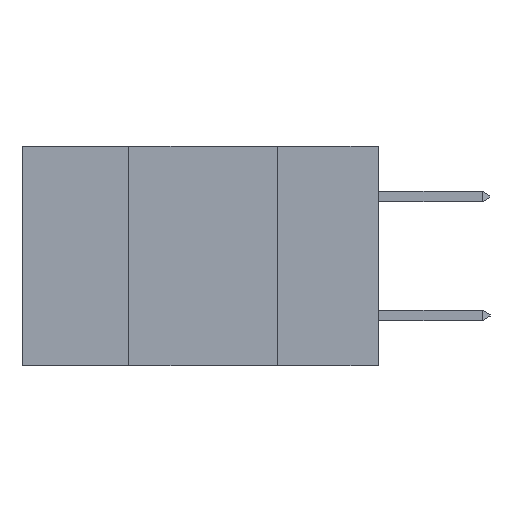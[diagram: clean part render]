
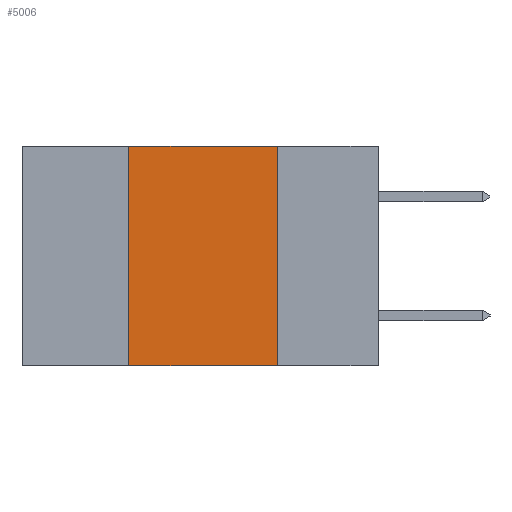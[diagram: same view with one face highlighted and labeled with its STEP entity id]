
A CAD part, left-side view. The second image highlights one B-rep face of the part: STEP entity #5006.
In plain terms, the highlighted planar face has unit normal (-1, 0, 0).
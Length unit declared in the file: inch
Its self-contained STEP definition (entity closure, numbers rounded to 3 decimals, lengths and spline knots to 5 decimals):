
#639 = CARTESIAN_POINT ( 'NONE',  ( 0., 0.17, 0. ) ) ;
#1431 = VECTOR ( 'NONE', #6552, 39.37008 ) ;
#1481 = DIRECTION ( 'NONE',  ( 0., -1., 0. ) ) ;
#1572 = CARTESIAN_POINT ( 'NONE',  ( 0., 0.42, -0.37 ) ) ;
#1961 = VERTEX_POINT ( 'NONE', #10551 ) ;
#2217 = ORIENTED_EDGE ( 'NONE', *, *, #4929, .T. ) ;
#2484 = CARTESIAN_POINT ( 'NONE',  ( 0., 0.17, -0.37 ) ) ;
#2720 = EDGE_CURVE ( 'NONE', #11193, #2944, #4649, .T. ) ;
#2770 = LINE ( 'NONE', #5174, #10688 ) ;
#2944 = VERTEX_POINT ( 'NONE', #2484 ) ;
#3335 = VERTEX_POINT ( 'NONE', #1572 ) ;
#3726 = CARTESIAN_POINT ( 'NONE',  ( 0., 0.42, -0.37 ) ) ;
#3785 = DIRECTION ( 'NONE',  ( 0., 0., -1. ) ) ;
#3831 = DIRECTION ( 'NONE',  ( 1., 0., 0. ) ) ;
#4030 = CARTESIAN_POINT ( 'NONE',  ( 0., 0.6, 0. ) ) ;
#4129 = PLANE ( 'NONE',  #8457 ) ;
#4649 = LINE ( 'NONE', #6662, #1431 ) ;
#4929 = EDGE_CURVE ( 'NONE', #3335, #2944, #2770, .T. ) ;
#4952 = DIRECTION ( 'NONE',  ( 0., -1., 0. ) ) ;
#5006 = ADVANCED_FACE ( 'NONE', ( #13049 ), #4129, .F. ) ;
#5174 = CARTESIAN_POINT ( 'NONE',  ( 0., 0.6, -0.37 ) ) ;
#6552 = DIRECTION ( 'NONE',  ( 0., 0., -1. ) ) ;
#6593 = VECTOR ( 'NONE', #11952, 39.37008 ) ;
#6662 = CARTESIAN_POINT ( 'NONE',  ( 0., 0.17, -0.37 ) ) ;
#7306 = VECTOR ( 'NONE', #1481, 39.37008 ) ;
#8457 = AXIS2_PLACEMENT_3D ( 'NONE', #4030, #3831, #3785 ) ;
#8822 = CARTESIAN_POINT ( 'NONE',  ( 0., 0.6, 0. ) ) ;
#9291 = LINE ( 'NONE', #3726, #6593 ) ;
#9820 = EDGE_CURVE ( 'NONE', #1961, #11193, #12464, .T. ) ;
#10148 = ORIENTED_EDGE ( 'NONE', *, *, #2720, .F. ) ;
#10278 = ORIENTED_EDGE ( 'NONE', *, *, #9820, .F. ) ;
#10551 = CARTESIAN_POINT ( 'NONE',  ( 0., 0.42, 0. ) ) ;
#10688 = VECTOR ( 'NONE', #4952, 39.37008 ) ;
#10907 = EDGE_LOOP ( 'NONE', ( #10148, #10278, #11958, #2217 ) ) ;
#11193 = VERTEX_POINT ( 'NONE', #639 ) ;
#11952 = DIRECTION ( 'NONE',  ( 0., 0., 1. ) ) ;
#11958 = ORIENTED_EDGE ( 'NONE', *, *, #13442, .F. ) ;
#12464 = LINE ( 'NONE', #8822, #7306 ) ;
#13049 = FACE_OUTER_BOUND ( 'NONE', #10907, .T. ) ;
#13442 = EDGE_CURVE ( 'NONE', #3335, #1961, #9291, .T. ) ;
